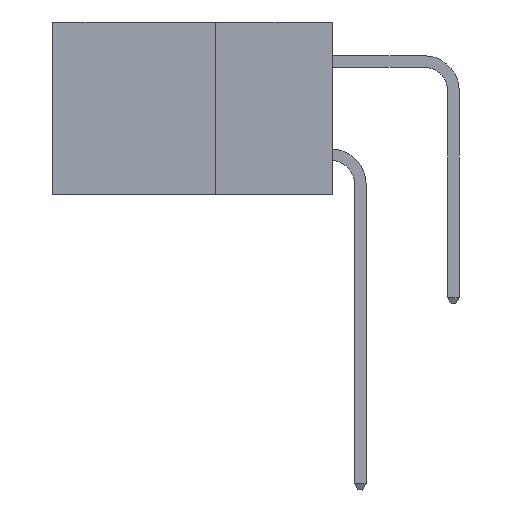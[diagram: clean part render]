
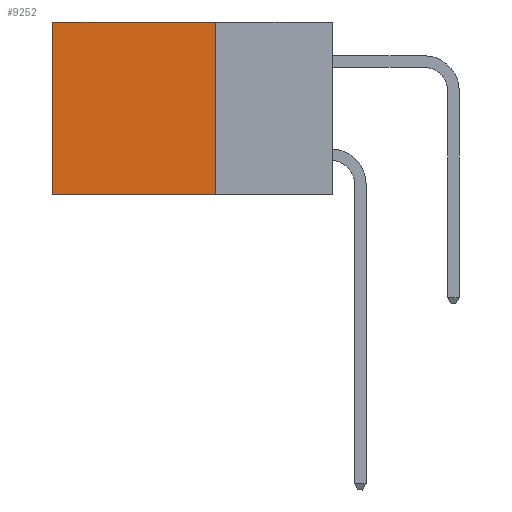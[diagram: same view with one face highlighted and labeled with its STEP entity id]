
A CAD part, left-side view. The second image highlights one B-rep face of the part: STEP entity #9252.
In plain terms, the highlighted planar face has unit normal (-1, 0, 0).
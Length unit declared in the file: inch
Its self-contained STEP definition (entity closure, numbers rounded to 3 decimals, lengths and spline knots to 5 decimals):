
#3680 = CARTESIAN_POINT ( 'NONE',  ( 0.298, 0.25, -0.37 ) ) ;
#4222 = LINE ( 'NONE', #21554, #32035 ) ;
#4240 = EDGE_CURVE ( 'NONE', #34795, #22979, #16928, .T. ) ;
#4389 = EDGE_CURVE ( 'NONE', #33779, #22979, #33769, .T. ) ;
#4915 = VERTEX_POINT ( 'NONE', #23149 ) ;
#4987 = EDGE_CURVE ( 'NONE', #4915, #34795, #6299, .T. ) ;
#5796 = ORIENTED_EDGE ( 'NONE', *, *, #4389, .F. ) ;
#5842 = VECTOR ( 'NONE', #34103, 39.37008 ) ;
#6299 = LINE ( 'NONE', #28761, #5842 ) ;
#6339 = VECTOR ( 'NONE', #29836, 39.37008 ) ;
#9252 = ADVANCED_FACE ( 'NONE', ( #33089 ), #34398, .F. ) ;
#10236 = CARTESIAN_POINT ( 'NONE',  ( 0.298, 0.6, 0. ) ) ;
#11193 = ORIENTED_EDGE ( 'NONE', *, *, #4240, .T. ) ;
#11768 = DIRECTION ( 'NONE',  ( 0., 0., -1. ) ) ;
#13619 = CARTESIAN_POINT ( 'NONE',  ( 0.298, 0.25, -0.37 ) ) ;
#16837 = EDGE_CURVE ( 'NONE', #4915, #33779, #4222, .T. ) ;
#16928 = LINE ( 'NONE', #25082, #33361 ) ;
#18203 = EDGE_LOOP ( 'NONE', ( #11193, #5796, #22869, #31010 ) ) ;
#18250 = DIRECTION ( 'NONE',  ( 0., 0., -1. ) ) ;
#21554 = CARTESIAN_POINT ( 'NONE',  ( 0.298, 0.25, 0. ) ) ;
#22859 = DIRECTION ( 'NONE',  ( 0., 0., -1. ) ) ;
#22869 = ORIENTED_EDGE ( 'NONE', *, *, #16837, .F. ) ;
#22979 = VERTEX_POINT ( 'NONE', #25361 ) ;
#23149 = CARTESIAN_POINT ( 'NONE',  ( 0.298, 0.25, 0. ) ) ;
#23424 = CARTESIAN_POINT ( 'NONE',  ( 0.298, 0.25, 0. ) ) ;
#25082 = CARTESIAN_POINT ( 'NONE',  ( 0.298, 0.6, 0. ) ) ;
#25361 = CARTESIAN_POINT ( 'NONE',  ( 0.298, 0.6, -0.37 ) ) ;
#28761 = CARTESIAN_POINT ( 'NONE',  ( 0.298, 0.25, 0. ) ) ;
#29836 = DIRECTION ( 'NONE',  ( 0., 1., 0. ) ) ;
#31010 = ORIENTED_EDGE ( 'NONE', *, *, #4987, .T. ) ;
#32035 = VECTOR ( 'NONE', #22859, 39.37008 ) ;
#32503 = AXIS2_PLACEMENT_3D ( 'NONE', #23424, #34631, #18250 ) ;
#33089 = FACE_OUTER_BOUND ( 'NONE', #18203, .T. ) ;
#33361 = VECTOR ( 'NONE', #11768, 39.37008 ) ;
#33769 = LINE ( 'NONE', #13619, #6339 ) ;
#33779 = VERTEX_POINT ( 'NONE', #3680 ) ;
#34103 = DIRECTION ( 'NONE',  ( 0., 1., 0. ) ) ;
#34398 = PLANE ( 'NONE',  #32503 ) ;
#34631 = DIRECTION ( 'NONE',  ( 1., 0., 0. ) ) ;
#34795 = VERTEX_POINT ( 'NONE', #10236 ) ;
